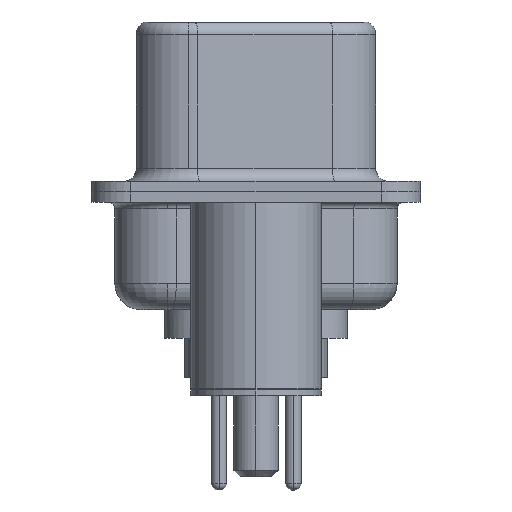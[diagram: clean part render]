
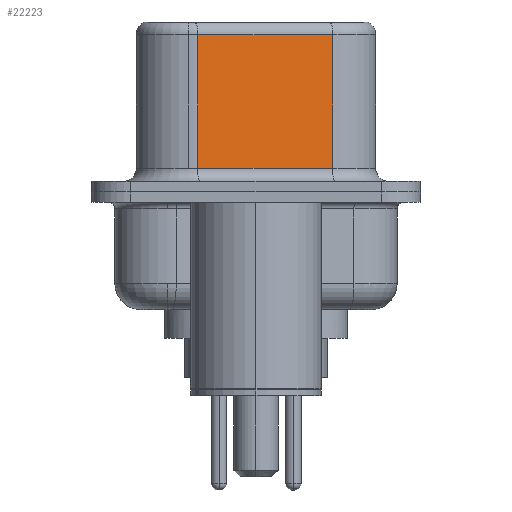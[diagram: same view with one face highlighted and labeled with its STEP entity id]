
A CAD part, left-side view. The second image highlights one B-rep face of the part: STEP entity #22223.
In plain terms, the highlighted planar face has unit normal (-0.985, -0.174, 0).
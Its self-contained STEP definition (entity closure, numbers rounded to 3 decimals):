
#24 = EDGE_CURVE ( 'NONE', #9727, #17212, #9265, .T. ) ;
#422 = CARTESIAN_POINT ( 'NONE',  ( 3.675, 2.233, 6.52 ) ) ;
#1012 = PLANE ( 'NONE',  #4059 ) ;
#1701 = VECTOR ( 'NONE', #14466, 1000. ) ;
#1783 = ORIENTED_EDGE ( 'NONE', *, *, #24, .F. ) ;
#3494 = VERTEX_POINT ( 'NONE', #7389 ) ;
#4059 = AXIS2_PLACEMENT_3D ( 'NONE', #4523, #16849, #6215 ) ;
#4453 = VERTEX_POINT ( 'NONE', #4943 ) ;
#4523 = CARTESIAN_POINT ( 'NONE',  ( 4.585, -2.927, 6.52 ) ) ;
#4620 = DIRECTION ( 'NONE',  ( 0., 0., -1. ) ) ;
#4943 = CARTESIAN_POINT ( 'NONE',  ( 3.675, 2.233, 0.9 ) ) ;
#5412 = VECTOR ( 'NONE', #16127, 1000. ) ;
#6215 = DIRECTION ( 'NONE',  ( -0.174, 0.985, 0. ) ) ;
#6458 = LINE ( 'NONE', #12504, #5412 ) ;
#6518 = CARTESIAN_POINT ( 'NONE',  ( 4.585, -2.927, 6.52 ) ) ;
#6792 = DIRECTION ( 'NONE',  ( 0.174, -0.985, 0. ) ) ;
#7389 = CARTESIAN_POINT ( 'NONE',  ( 3.675, 2.233, 6.02 ) ) ;
#9265 = LINE ( 'NONE', #6518, #17694 ) ;
#9727 = VERTEX_POINT ( 'NONE', #13562 ) ;
#10124 = CARTESIAN_POINT ( 'NONE',  ( 4.585, -2.927, 0.9 ) ) ;
#10275 = EDGE_LOOP ( 'NONE', ( #1783, #16624, #15277, #13780 ) ) ;
#10323 = CARTESIAN_POINT ( 'NONE',  ( 4.585, -2.927, 0.9 ) ) ;
#12504 = CARTESIAN_POINT ( 'NONE',  ( 4.585, -2.927, 6.02 ) ) ;
#13562 = CARTESIAN_POINT ( 'NONE',  ( 4.585, -2.927, 6.02 ) ) ;
#13780 = ORIENTED_EDGE ( 'NONE', *, *, #16725, .T. ) ;
#14466 = DIRECTION ( 'NONE',  ( 0., 0., -1. ) ) ;
#14815 = EDGE_CURVE ( 'NONE', #3494, #4453, #20766, .T. ) ;
#14845 = LINE ( 'NONE', #10323, #19419 ) ;
#15277 = ORIENTED_EDGE ( 'NONE', *, *, #14815, .T. ) ;
#16127 = DIRECTION ( 'NONE',  ( -0.174, 0.985, 0. ) ) ;
#16624 = ORIENTED_EDGE ( 'NONE', *, *, #20047, .T. ) ;
#16725 = EDGE_CURVE ( 'NONE', #4453, #17212, #14845, .T. ) ;
#16849 = DIRECTION ( 'NONE',  ( 0.985, 0.174, 0. ) ) ;
#17212 = VERTEX_POINT ( 'NONE', #10124 ) ;
#17694 = VECTOR ( 'NONE', #4620, 1000. ) ;
#18295 = FACE_OUTER_BOUND ( 'NONE', #10275, .T. ) ;
#19419 = VECTOR ( 'NONE', #6792, 1000. ) ;
#20047 = EDGE_CURVE ( 'NONE', #9727, #3494, #6458, .T. ) ;
#20766 = LINE ( 'NONE', #422, #1701 ) ;
#22223 = ADVANCED_FACE ( 'NONE', ( #18295 ), #1012, .F. ) ;
